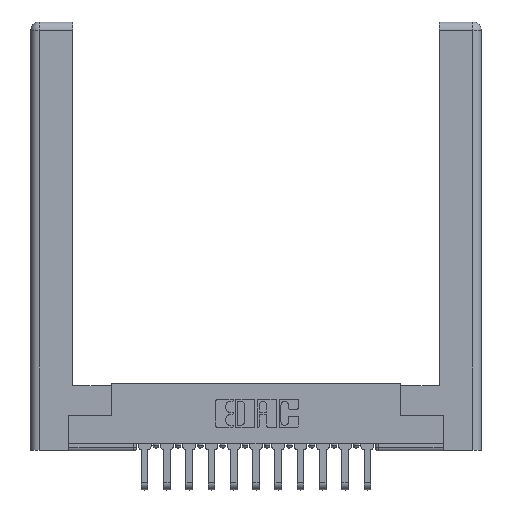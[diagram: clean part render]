
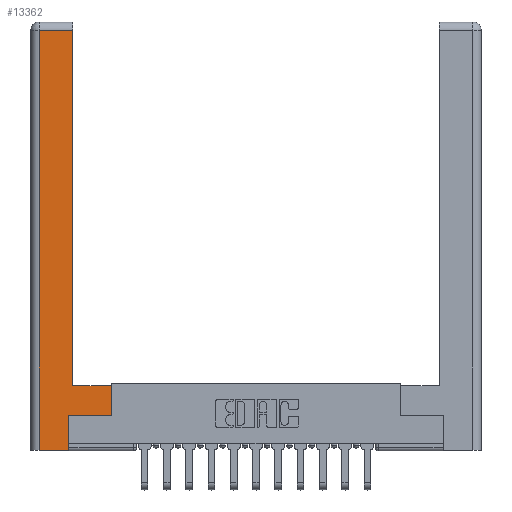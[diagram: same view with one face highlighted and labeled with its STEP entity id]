
A CAD part, top view. The second image highlights one B-rep face of the part: STEP entity #13362.
In plain terms, the highlighted planar face has unit normal (0, 0, 1).
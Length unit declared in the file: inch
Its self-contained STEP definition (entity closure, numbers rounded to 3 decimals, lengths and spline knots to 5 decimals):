
#115 = LINE ( 'NONE', #2488, #497 ) ;
#295 = VERTEX_POINT ( 'NONE', #14450 ) ;
#416 = CARTESIAN_POINT ( 'NONE',  ( 0.295, 3., 0. ) ) ;
#474 = FACE_OUTER_BOUND ( 'NONE', #10381, .T. ) ;
#497 = VECTOR ( 'NONE', #5081, 39.37008 ) ;
#755 = EDGE_CURVE ( 'NONE', #15451, #2760, #1741, .T. ) ;
#1583 = VERTEX_POINT ( 'NONE', #5773 ) ;
#1663 = DIRECTION ( 'NONE',  ( 0., 0., -1. ) ) ;
#1741 = LINE ( 'NONE', #1916, #5027 ) ;
#1821 = DIRECTION ( 'NONE',  ( -1., 0., 0. ) ) ;
#1916 = CARTESIAN_POINT ( 'NONE',  ( 0.0615, 0., 0. ) ) ;
#1917 = LINE ( 'NONE', #4758, #3455 ) ;
#2027 = DIRECTION ( 'NONE',  ( 0., -1., 0. ) ) ;
#2042 = CARTESIAN_POINT ( 'NONE',  ( 0.0615, 2.94, 0. ) ) ;
#2076 = VECTOR ( 'NONE', #12027, 39.37008 ) ;
#2488 = CARTESIAN_POINT ( 'NONE',  ( 0.0615, 2.94, 0. ) ) ;
#2760 = VERTEX_POINT ( 'NONE', #6385 ) ;
#3320 = LINE ( 'NONE', #13956, #13214 ) ;
#3455 = VECTOR ( 'NONE', #10902, 39.37008 ) ;
#3656 = CARTESIAN_POINT ( 'NONE',  ( 0.265, 0.245, 0. ) ) ;
#3719 = EDGE_CURVE ( 'NONE', #295, #11947, #7887, .T. ) ;
#4125 = DIRECTION ( 'NONE',  ( 0., 1., 0. ) ) ;
#4561 = VERTEX_POINT ( 'NONE', #14600 ) ;
#4739 = ORIENTED_EDGE ( 'NONE', *, *, #3719, .T. ) ;
#4758 = CARTESIAN_POINT ( 'NONE',  ( 0.565, 0.245, 0. ) ) ;
#5027 = VECTOR ( 'NONE', #2027, 39.37008 ) ;
#5073 = ORIENTED_EDGE ( 'NONE', *, *, #15215, .T. ) ;
#5081 = DIRECTION ( 'NONE',  ( -1., 0., 0. ) ) ;
#5187 = ORIENTED_EDGE ( 'NONE', *, *, #755, .T. ) ;
#5449 = EDGE_CURVE ( 'NONE', #8838, #15451, #115, .T. ) ;
#5773 = CARTESIAN_POINT ( 'NONE',  ( 0.565, 0.245, 0. ) ) ;
#6086 = LINE ( 'NONE', #416, #12102 ) ;
#6107 = EDGE_CURVE ( 'NONE', #4561, #8838, #6086, .T. ) ;
#6147 = ORIENTED_EDGE ( 'NONE', *, *, #6107, .T. ) ;
#6241 = CARTESIAN_POINT ( 'NONE',  ( 0.265, 0.245, 0. ) ) ;
#6385 = CARTESIAN_POINT ( 'NONE',  ( 0.0615, 0., 0. ) ) ;
#6531 = VECTOR ( 'NONE', #15295, 39.37008 ) ;
#6809 = PLANE ( 'NONE',  #7928 ) ;
#7791 = VECTOR ( 'NONE', #13119, 39.37008 ) ;
#7887 = LINE ( 'NONE', #6241, #2076 ) ;
#7928 = AXIS2_PLACEMENT_3D ( 'NONE', #11628, #1663, #9117 ) ;
#8838 = VERTEX_POINT ( 'NONE', #13859 ) ;
#9117 = DIRECTION ( 'NONE',  ( -1., 0., 0. ) ) ;
#10001 = ORIENTED_EDGE ( 'NONE', *, *, #14708, .T. ) ;
#10381 = EDGE_LOOP ( 'NONE', ( #6147, #13580, #5187, #10001, #4739, #13694, #11500, #5073 ) ) ;
#10902 = DIRECTION ( 'NONE',  ( 1., 0., 0. ) ) ;
#11239 = EDGE_CURVE ( 'NONE', #11947, #1583, #1917, .T. ) ;
#11500 = ORIENTED_EDGE ( 'NONE', *, *, #11680, .T. ) ;
#11628 = CARTESIAN_POINT ( 'NONE',  ( 0., 0., 0. ) ) ;
#11680 = EDGE_CURVE ( 'NONE', #1583, #14619, #12944, .T. ) ;
#11947 = VERTEX_POINT ( 'NONE', #3656 ) ;
#12027 = DIRECTION ( 'NONE',  ( 0., 1., 0. ) ) ;
#12102 = VECTOR ( 'NONE', #4125, 39.37008 ) ;
#12779 = CARTESIAN_POINT ( 'NONE',  ( 0.565, 0.45, 0. ) ) ;
#12944 = LINE ( 'NONE', #13045, #6531 ) ;
#13045 = CARTESIAN_POINT ( 'NONE',  ( 0.565, 0.45, 0. ) ) ;
#13119 = DIRECTION ( 'NONE',  ( 1., 0., 0. ) ) ;
#13214 = VECTOR ( 'NONE', #1821, 39.37008 ) ;
#13362 = ADVANCED_FACE ( 'NONE', ( #474 ), #6809, .F. ) ;
#13580 = ORIENTED_EDGE ( 'NONE', *, *, #5449, .T. ) ;
#13694 = ORIENTED_EDGE ( 'NONE', *, *, #11239, .T. ) ;
#13859 = CARTESIAN_POINT ( 'NONE',  ( 0.295, 2.94, 0. ) ) ;
#13956 = CARTESIAN_POINT ( 'NONE',  ( 0.295, 0.45, 0. ) ) ;
#14175 = CARTESIAN_POINT ( 'NONE',  ( 0.265, 0., 0. ) ) ;
#14450 = CARTESIAN_POINT ( 'NONE',  ( 0.265, 0., 0. ) ) ;
#14600 = CARTESIAN_POINT ( 'NONE',  ( 0.295, 0.45, 0. ) ) ;
#14619 = VERTEX_POINT ( 'NONE', #12779 ) ;
#14708 = EDGE_CURVE ( 'NONE', #2760, #295, #15698, .T. ) ;
#15215 = EDGE_CURVE ( 'NONE', #14619, #4561, #3320, .T. ) ;
#15295 = DIRECTION ( 'NONE',  ( 0., 1., 0. ) ) ;
#15451 = VERTEX_POINT ( 'NONE', #2042 ) ;
#15698 = LINE ( 'NONE', #14175, #7791 ) ;
